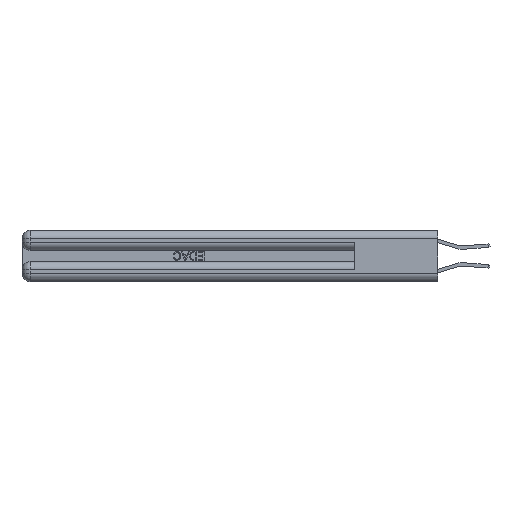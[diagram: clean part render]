
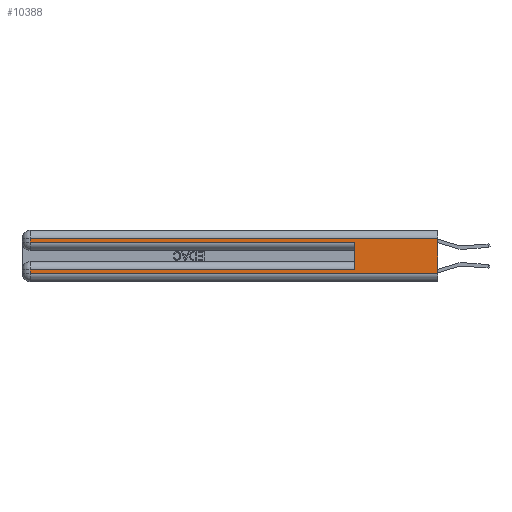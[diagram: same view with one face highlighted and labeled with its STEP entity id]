
A CAD part, left-side view. The second image highlights one B-rep face of the part: STEP entity #10388.
In plain terms, the highlighted planar face has unit normal (-1, 0, 0).
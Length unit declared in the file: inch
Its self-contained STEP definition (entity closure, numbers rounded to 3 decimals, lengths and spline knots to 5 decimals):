
#207 = EDGE_CURVE ( 'NONE', #16596, #24995, #7369, .T. ) ;
#240 = VECTOR ( 'NONE', #3982, 39.37008 ) ;
#563 = CARTESIAN_POINT ( 'NONE',  ( 0., 0.6, 0.285 ) ) ;
#614 = DIRECTION ( 'NONE',  ( 0., 0., -1. ) ) ;
#1561 = ORIENTED_EDGE ( 'NONE', *, *, #20843, .T. ) ;
#2979 = PLANE ( 'NONE',  #19707 ) ;
#3805 = CARTESIAN_POINT ( 'NONE',  ( 0., 2.94, 0.37 ) ) ;
#3982 = DIRECTION ( 'NONE',  ( 0., 0., -1. ) ) ;
#4377 = ORIENTED_EDGE ( 'NONE', *, *, #7720, .T. ) ;
#4416 = CARTESIAN_POINT ( 'NONE',  ( 0., 0., 0.31 ) ) ;
#4534 = EDGE_CURVE ( 'NONE', #6291, #17491, #19026, .T. ) ;
#4761 = ORIENTED_EDGE ( 'NONE', *, *, #17258, .T. ) ;
#6075 = LINE ( 'NONE', #17741, #16344 ) ;
#6100 = ORIENTED_EDGE ( 'NONE', *, *, #25295, .T. ) ;
#6223 = VECTOR ( 'NONE', #18492, 39.37008 ) ;
#6291 = VERTEX_POINT ( 'NONE', #18751 ) ;
#6542 = CARTESIAN_POINT ( 'NONE',  ( 0., 2.94, 0.285 ) ) ;
#6725 = DIRECTION ( 'NONE',  ( 0., 1., 0. ) ) ;
#7369 = LINE ( 'NONE', #27914, #20410 ) ;
#7720 = EDGE_CURVE ( 'NONE', #11472, #16596, #28041, .T. ) ;
#8788 = VECTOR ( 'NONE', #6725, 39.37008 ) ;
#10388 = ADVANCED_FACE ( 'NONE', ( #16149 ), #2979, .F. ) ;
#10495 = DIRECTION ( 'NONE',  ( 0., 1., 0. ) ) ;
#10640 = LINE ( 'NONE', #3805, #15819 ) ;
#10652 = EDGE_CURVE ( 'NONE', #24995, #17491, #23031, .T. ) ;
#11009 = EDGE_CURVE ( 'NONE', #11472, #21873, #27174, .T. ) ;
#11403 = ORIENTED_EDGE ( 'NONE', *, *, #10652, .T. ) ;
#11472 = VERTEX_POINT ( 'NONE', #25503 ) ;
#11890 = CARTESIAN_POINT ( 'NONE',  ( 0., 0., 0.37 ) ) ;
#12412 = CARTESIAN_POINT ( 'NONE',  ( 0., 0., 0.085 ) ) ;
#12991 = LINE ( 'NONE', #12412, #19913 ) ;
#15819 = VECTOR ( 'NONE', #17132, 39.37008 ) ;
#16149 = FACE_OUTER_BOUND ( 'NONE', #18378, .T. ) ;
#16344 = VECTOR ( 'NONE', #26503, 39.37008 ) ;
#16596 = VERTEX_POINT ( 'NONE', #21394 ) ;
#17117 = CARTESIAN_POINT ( 'NONE',  ( 0., 0., 0.37 ) ) ;
#17132 = DIRECTION ( 'NONE',  ( 0., 0., -1. ) ) ;
#17258 = EDGE_CURVE ( 'NONE', #25666, #24147, #10640, .T. ) ;
#17491 = VERTEX_POINT ( 'NONE', #563 ) ;
#17629 = CARTESIAN_POINT ( 'NONE',  ( 0., 2.94, 0.085 ) ) ;
#17741 = CARTESIAN_POINT ( 'NONE',  ( 0., 0., 0.06 ) ) ;
#18378 = EDGE_LOOP ( 'NONE', ( #23974, #4377, #20393, #11403, #27681, #6100, #4761, #1561 ) ) ;
#18391 = CARTESIAN_POINT ( 'NONE',  ( 0., 0., 0.285 ) ) ;
#18492 = DIRECTION ( 'NONE',  ( 0., -1., 0. ) ) ;
#18751 = CARTESIAN_POINT ( 'NONE',  ( 0., 0.6, 0.085 ) ) ;
#19026 = LINE ( 'NONE', #23479, #20067 ) ;
#19707 = AXIS2_PLACEMENT_3D ( 'NONE', #11890, #24905, #614 ) ;
#19913 = VECTOR ( 'NONE', #10495, 39.37008 ) ;
#20067 = VECTOR ( 'NONE', #26101, 39.37008 ) ;
#20393 = ORIENTED_EDGE ( 'NONE', *, *, #207, .T. ) ;
#20410 = VECTOR ( 'NONE', #23758, 39.37008 ) ;
#20843 = EDGE_CURVE ( 'NONE', #24147, #21873, #6075, .T. ) ;
#21394 = CARTESIAN_POINT ( 'NONE',  ( 0., 2.94, 0.31 ) ) ;
#21873 = VERTEX_POINT ( 'NONE', #28431 ) ;
#23031 = LINE ( 'NONE', #18391, #6223 ) ;
#23479 = CARTESIAN_POINT ( 'NONE',  ( 0., 0.6, 0.145 ) ) ;
#23758 = DIRECTION ( 'NONE',  ( 0., 0., -1. ) ) ;
#23834 = CARTESIAN_POINT ( 'NONE',  ( 0., 2.94, 0.06 ) ) ;
#23974 = ORIENTED_EDGE ( 'NONE', *, *, #11009, .F. ) ;
#24147 = VERTEX_POINT ( 'NONE', #23834 ) ;
#24905 = DIRECTION ( 'NONE',  ( 1., 0., 0. ) ) ;
#24995 = VERTEX_POINT ( 'NONE', #6542 ) ;
#25295 = EDGE_CURVE ( 'NONE', #6291, #25666, #12991, .T. ) ;
#25503 = CARTESIAN_POINT ( 'NONE',  ( 0., 0., 0.31 ) ) ;
#25666 = VERTEX_POINT ( 'NONE', #17629 ) ;
#26101 = DIRECTION ( 'NONE',  ( 0., 0., 1. ) ) ;
#26503 = DIRECTION ( 'NONE',  ( 0., -1., 0. ) ) ;
#27174 = LINE ( 'NONE', #17117, #240 ) ;
#27681 = ORIENTED_EDGE ( 'NONE', *, *, #4534, .F. ) ;
#27914 = CARTESIAN_POINT ( 'NONE',  ( 0., 2.94, 0.37 ) ) ;
#28041 = LINE ( 'NONE', #4416, #8788 ) ;
#28431 = CARTESIAN_POINT ( 'NONE',  ( 0., 0., 0.06 ) ) ;
